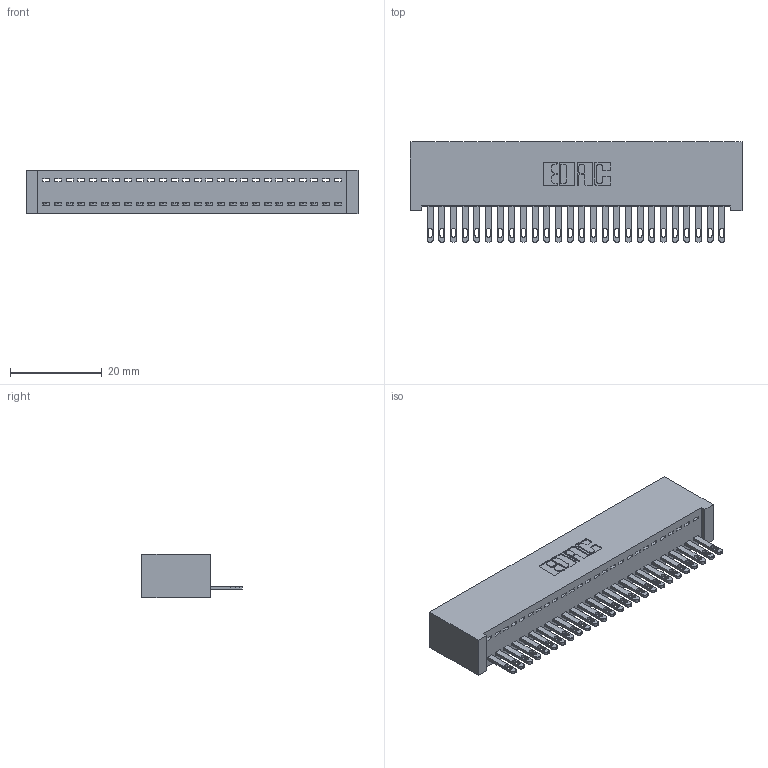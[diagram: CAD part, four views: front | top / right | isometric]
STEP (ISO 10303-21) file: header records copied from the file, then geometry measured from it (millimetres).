
FILE_DESCRIPTION (( 'STEP AP203' ), '1' );
FILE_NAME ('892-026-500-101.STEP', '2020-09-21T14:34:12', ( '' ), ( '' ), 'SwSTEP 2.0', 'SolidWorks 2020', '' );
FILE_SCHEMA (( 'CONFIG_CONTROL_DESIGN' ));
Length unit declared in the file: inch
Products named in the file (3): 892-026-500-101; 842 Part_Lugless; 345-292-001_345-293-100
Assembly tree (27 placements, depth 2):
  892-026-500-101
    842 Part_Lugless
    345-292-001_345-293-100  x26
Bounding box: 72.29 x 21.85 x 9.4 mm (x, y, z)
Volume: 6704.4 mm3; surface area: 9920.8 mm2
Topology: 27 solids, 27 shells, 1506 faces, 4643 edges, 3094 vertices
Faces by surface type: plane 998, cylinder 508
Entity records: 17485 total; most frequent: CARTESIAN_POINT 3024, ORIENTED_EDGE 2986, DIRECTION 2577, EDGE_CURVE 1493, VECTOR 1369, LINE 1369, VERTEX_POINT 994, AXIS2_PLACEMENT_3D 604
